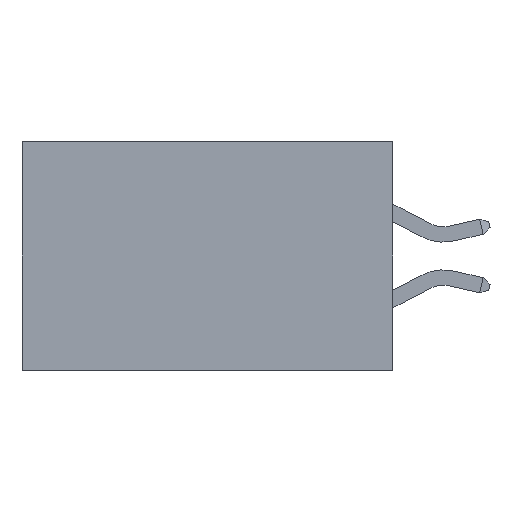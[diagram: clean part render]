
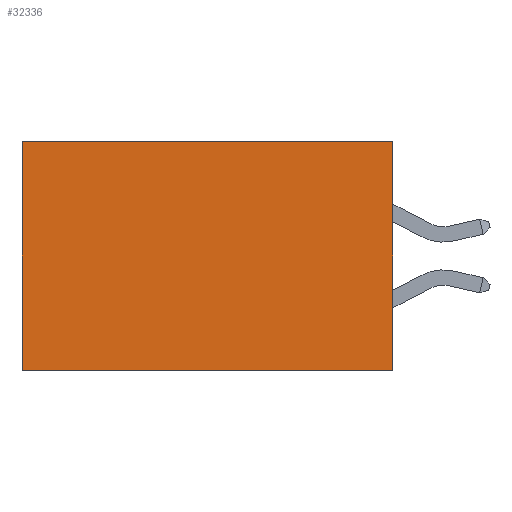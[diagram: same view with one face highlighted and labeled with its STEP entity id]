
A CAD part, left-side view. The second image highlights one B-rep face of the part: STEP entity #32336.
In plain terms, the highlighted planar face has unit normal (-1, 0, 0).
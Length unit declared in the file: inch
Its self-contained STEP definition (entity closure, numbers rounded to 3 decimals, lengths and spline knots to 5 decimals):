
#938 = DIRECTION ( 'NONE',  ( 0., 0., -1. ) ) ;
#1335 = DIRECTION ( 'NONE',  ( 1., 0., 0. ) ) ;
#1375 = CARTESIAN_POINT ( 'NONE',  ( 0.2875, 0.6, -0.37 ) ) ;
#1493 = DIRECTION ( 'NONE',  ( 0., 1., 0. ) ) ;
#2123 = LINE ( 'NONE', #12162, #18786 ) ;
#2805 = EDGE_CURVE ( 'NONE', #29249, #15475, #26175, .T. ) ;
#3136 = DIRECTION ( 'NONE',  ( 0., 0., -1. ) ) ;
#4770 = VERTEX_POINT ( 'NONE', #14384 ) ;
#6042 = PLANE ( 'NONE',  #21495 ) ;
#6093 = LINE ( 'NONE', #24364, #21904 ) ;
#6145 = DIRECTION ( 'NONE',  ( 0., 0., -1. ) ) ;
#6243 = EDGE_CURVE ( 'NONE', #24652, #15475, #6093, .T. ) ;
#9202 = ORIENTED_EDGE ( 'NONE', *, *, #2805, .T. ) ;
#10666 = EDGE_CURVE ( 'NONE', #4770, #29249, #2123, .T. ) ;
#11650 = FACE_OUTER_BOUND ( 'NONE', #32186, .T. ) ;
#12162 = CARTESIAN_POINT ( 'NONE',  ( 0.2875, 0., 0. ) ) ;
#14384 = CARTESIAN_POINT ( 'NONE',  ( 0.2875, 0., 0. ) ) ;
#14693 = LINE ( 'NONE', #31546, #27191 ) ;
#15280 = VECTOR ( 'NONE', #938, 39.37008 ) ;
#15475 = VERTEX_POINT ( 'NONE', #1375 ) ;
#16407 = EDGE_CURVE ( 'NONE', #4770, #24652, #14693, .T. ) ;
#16906 = CARTESIAN_POINT ( 'NONE',  ( 0.2875, 0., 0. ) ) ;
#18786 = VECTOR ( 'NONE', #1493, 39.37008 ) ;
#20779 = ORIENTED_EDGE ( 'NONE', *, *, #6243, .F. ) ;
#21495 = AXIS2_PLACEMENT_3D ( 'NONE', #16906, #1335, #6145 ) ;
#21904 = VECTOR ( 'NONE', #32605, 39.37008 ) ;
#23437 = CARTESIAN_POINT ( 'NONE',  ( 0.2875, 0.6, 0. ) ) ;
#24364 = CARTESIAN_POINT ( 'NONE',  ( 0.2875, 0., -0.37 ) ) ;
#24652 = VERTEX_POINT ( 'NONE', #32967 ) ;
#26175 = LINE ( 'NONE', #29122, #15280 ) ;
#27191 = VECTOR ( 'NONE', #3136, 39.37008 ) ;
#29122 = CARTESIAN_POINT ( 'NONE',  ( 0.2875, 0.6, 0. ) ) ;
#29249 = VERTEX_POINT ( 'NONE', #23437 ) ;
#29703 = ORIENTED_EDGE ( 'NONE', *, *, #10666, .T. ) ;
#31546 = CARTESIAN_POINT ( 'NONE',  ( 0.2875, 0., 0. ) ) ;
#32186 = EDGE_LOOP ( 'NONE', ( #9202, #20779, #32429, #29703 ) ) ;
#32336 = ADVANCED_FACE ( 'NONE', ( #11650 ), #6042, .F. ) ;
#32429 = ORIENTED_EDGE ( 'NONE', *, *, #16407, .F. ) ;
#32605 = DIRECTION ( 'NONE',  ( 0., 1., 0. ) ) ;
#32967 = CARTESIAN_POINT ( 'NONE',  ( 0.2875, 0., -0.37 ) ) ;
